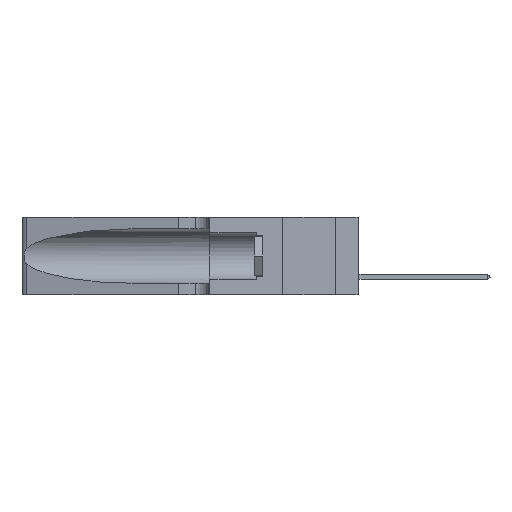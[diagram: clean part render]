
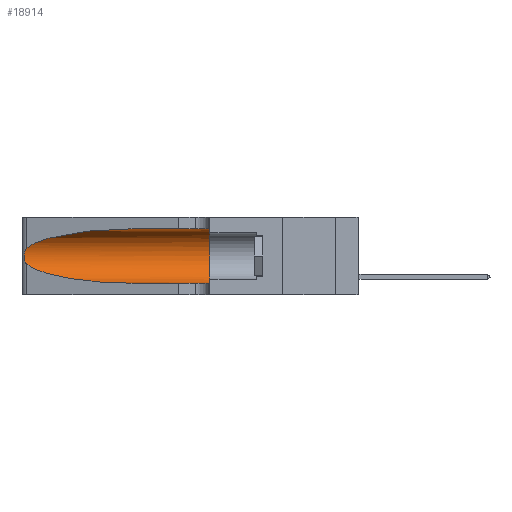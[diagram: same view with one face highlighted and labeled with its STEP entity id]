
A CAD part, left-side view. The second image highlights one B-rep face of the part: STEP entity #18914.
In plain terms, the highlighted cylindrical face has radius 3.308 mm (diameter 6.617 mm), a partial arc.
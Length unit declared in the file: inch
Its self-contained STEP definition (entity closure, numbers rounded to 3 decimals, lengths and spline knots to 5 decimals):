
#1822 = ORIENTED_EDGE ( 'NONE', *, *, #13658, .T. ) ;
#2249 = ORIENTED_EDGE ( 'NONE', *, *, #10633, .T. ) ;
#2755 = CARTESIAN_POINT ( 'NONE',  ( 0.25487, 1.22718, 0.22369 ) ) ;
#2775 = VERTEX_POINT ( 'NONE', #5705 ) ;
#2811 = CARTESIAN_POINT ( 'NONE',  ( 0.26018, 1.23835, 0.19895 ) ) ;
#3400 = CARTESIAN_POINT ( 'NONE',  ( 0.25487, 1.22718, 0.14631 ) ) ;
#3680 = CARTESIAN_POINT ( 'NONE',  ( 0.1305, 0.72297, 0.31525 ) ) ;
#4207 = DIRECTION ( 'NONE',  ( 0., -1., 0. ) ) ;
#4311 = ORIENTED_EDGE ( 'NONE', *, *, #23033, .F. ) ;
#4325 = CARTESIAN_POINT ( 'NONE',  ( 0.25487, 1.22718, 0.22369 ) ) ;
#5035 = CARTESIAN_POINT ( 'NONE',  ( 0.18966, 0.96281, 0.31525 ) ) ;
#5705 = CARTESIAN_POINT ( 'NONE',  ( 0.25487, 1.22718, 0.22369 ) ) ;
#5867 = EDGE_CURVE ( 'NONE', #16106, #2775, #28144, .T. ) ;
#6275 = CARTESIAN_POINT ( 'NONE',  ( 0.1305, 0.35, 0.31525 ) ) ;
#6606 = CARTESIAN_POINT ( 'NONE',  ( 0.1305, 1.61858, 0.31525 ) ) ;
#6843 = CARTESIAN_POINT ( 'NONE',  ( 0.1305, 0.72297, 0.31525 ) ) ;
#7094 = CARTESIAN_POINT ( 'NONE',  ( 0.1305, 1.61858, 0.185 ) ) ;
#7624 = DIRECTION ( 'NONE',  ( 0., 0., 1. ) ) ;
#7910 = CARTESIAN_POINT ( 'NONE',  ( 0.18966, 0.96281, 0.05475 ) ) ;
#8724 = ORIENTED_EDGE ( 'NONE', *, *, #16446, .F. ) ;
#9929 = CARTESIAN_POINT ( 'NONE',  ( 0.2373, 1.15595, 0.28018 ) ) ;
#10548 =( BOUNDED_CURVE ( )  B_SPLINE_CURVE ( 3, ( #17319, #22203, #7910, #12742 ),
 .UNSPECIFIED., .F., .T. ) 
 B_SPLINE_CURVE_WITH_KNOTS ( ( 4, 4 ),
 ( 3.44316, 4.71239 ),
 .UNSPECIFIED. ) 
 CURVE ( )  GEOMETRIC_REPRESENTATION_ITEM ( )  RATIONAL_B_SPLINE_CURVE ( ( 1., 0.87, 0.87, 1. ) ) 
 REPRESENTATION_ITEM ( '' )  );
#10633 = EDGE_CURVE ( 'NONE', #23481, #18926, #10548, .T. ) ;
#11854 = DIRECTION ( 'NONE',  ( 0., 1., 0. ) ) ;
#12645 = VECTOR ( 'NONE', #20449, 39.37008 ) ;
#12742 = CARTESIAN_POINT ( 'NONE',  ( 0.1305, 0.72297, 0.05475 ) ) ;
#13242 = B_SPLINE_CURVE_WITH_KNOTS ( 'NONE', 3,
 ( #4325, #25859, #16892, #19617, #14657, #2811, #27067, #13734, #21726, #24549, #24659, #27020, #17576, #3400 ),
 .UNSPECIFIED., .F., .F.,
 ( 4, 2, 2, 2, 2, 2, 4 ),
 ( 0., 0.00027, 0.00053, 0.00107, 0.0016, 0.00187, 0.00214 ),
 .UNSPECIFIED. ) ;
#13658 = EDGE_CURVE ( 'NONE', #2775, #23481, #13242, .T. ) ;
#13734 = CARTESIAN_POINT ( 'NONE',  ( 0.26075, 1.23896, 0.178 ) ) ;
#14516 = VERTEX_POINT ( 'NONE', #6275 ) ;
#14522 = CARTESIAN_POINT ( 'NONE',  ( 0.1305, 0.35, 0.185 ) ) ;
#14652 = ORIENTED_EDGE ( 'NONE', *, *, #27772, .T. ) ;
#14657 = CARTESIAN_POINT ( 'NONE',  ( 0.25854, 1.2359, 0.20912 ) ) ;
#16018 = LINE ( 'NONE', #18709, #29073 ) ;
#16106 = VERTEX_POINT ( 'NONE', #3680 ) ;
#16446 = EDGE_CURVE ( 'NONE', #14516, #21482, #20885, .T. ) ;
#16892 = CARTESIAN_POINT ( 'NONE',  ( 0.25639, 1.23184, 0.21858 ) ) ;
#17319 = CARTESIAN_POINT ( 'NONE',  ( 0.25487, 1.22718, 0.14631 ) ) ;
#17576 = CARTESIAN_POINT ( 'NONE',  ( 0.25555, 1.22993, 0.14849 ) ) ;
#18709 = CARTESIAN_POINT ( 'NONE',  ( 0.1305, 1.61858, 0.05475 ) ) ;
#18914 = ADVANCED_FACE ( 'NONE', ( #22164 ), #20313, .F. ) ;
#18926 = VERTEX_POINT ( 'NONE', #25794 ) ;
#18971 = AXIS2_PLACEMENT_3D ( 'NONE', #7094, #23964, #21966 ) ;
#19531 = EDGE_LOOP ( 'NONE', ( #26073, #1822, #2249, #14652, #8724, #4311 ) ) ;
#19617 = CARTESIAN_POINT ( 'NONE',  ( 0.25787, 1.23484, 0.2124 ) ) ;
#20313 = CYLINDRICAL_SURFACE ( 'NONE', #18971, 0.13025 ) ;
#20380 = CARTESIAN_POINT ( 'NONE',  ( 0.1305, 0.35, 0.05475 ) ) ;
#20449 = DIRECTION ( 'NONE',  ( 0., -1., 0. ) ) ;
#20469 = LINE ( 'NONE', #6606, #12645 ) ;
#20885 = CIRCLE ( 'NONE', #29466, 0.13025 ) ;
#21482 = VERTEX_POINT ( 'NONE', #20380 ) ;
#21726 = CARTESIAN_POINT ( 'NONE',  ( 0.26017, 1.23833, 0.17102 ) ) ;
#21966 = DIRECTION ( 'NONE',  ( 0., 0., -1. ) ) ;
#22164 = FACE_OUTER_BOUND ( 'NONE', #19531, .T. ) ;
#22203 = CARTESIAN_POINT ( 'NONE',  ( 0.2373, 1.15595, 0.08982 ) ) ;
#23033 = EDGE_CURVE ( 'NONE', #16106, #14516, #20469, .T. ) ;
#23481 = VERTEX_POINT ( 'NONE', #24129 ) ;
#23964 = DIRECTION ( 'NONE',  ( 0., -1., 0. ) ) ;
#24129 = CARTESIAN_POINT ( 'NONE',  ( 0.25487, 1.22718, 0.14631 ) ) ;
#24549 = CARTESIAN_POINT ( 'NONE',  ( 0.25856, 1.23593, 0.16098 ) ) ;
#24659 = CARTESIAN_POINT ( 'NONE',  ( 0.25789, 1.23486, 0.15765 ) ) ;
#25794 = CARTESIAN_POINT ( 'NONE',  ( 0.1305, 0.72297, 0.05475 ) ) ;
#25859 = CARTESIAN_POINT ( 'NONE',  ( 0.25555, 1.22994, 0.2215 ) ) ;
#26073 = ORIENTED_EDGE ( 'NONE', *, *, #5867, .T. ) ;
#27020 = CARTESIAN_POINT ( 'NONE',  ( 0.25639, 1.23186, 0.15144 ) ) ;
#27067 = CARTESIAN_POINT ( 'NONE',  ( 0.26075, 1.23896, 0.19203 ) ) ;
#27772 = EDGE_CURVE ( 'NONE', #18926, #21482, #16018, .T. ) ;
#28144 =( BOUNDED_CURVE ( )  B_SPLINE_CURVE ( 3, ( #6843, #5035, #9929, #2755 ),
 .UNSPECIFIED., .F., .T. ) 
 B_SPLINE_CURVE_WITH_KNOTS ( ( 4, 4 ),
 ( 1.5708, 2.84003 ),
 .UNSPECIFIED. ) 
 CURVE ( )  GEOMETRIC_REPRESENTATION_ITEM ( )  RATIONAL_B_SPLINE_CURVE ( ( 1., 0.87, 0.87, 1. ) ) 
 REPRESENTATION_ITEM ( '' )  );
#29073 = VECTOR ( 'NONE', #4207, 39.37008 ) ;
#29466 = AXIS2_PLACEMENT_3D ( 'NONE', #14522, #11854, #7624 ) ;
